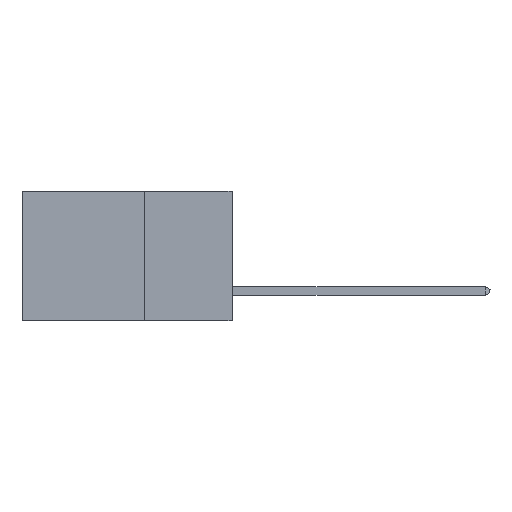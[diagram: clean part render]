
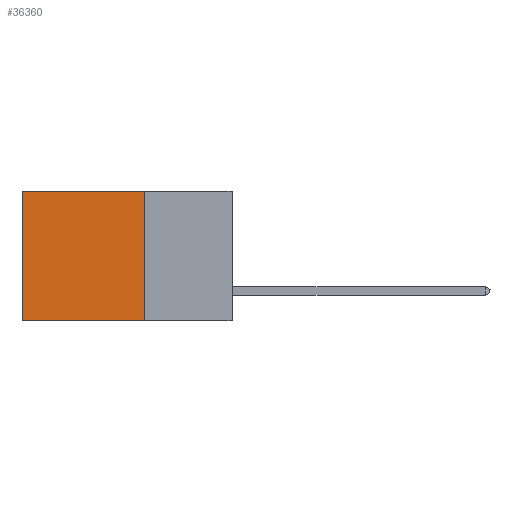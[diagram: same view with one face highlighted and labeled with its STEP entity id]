
A CAD part, left-side view. The second image highlights one B-rep face of the part: STEP entity #36360.
In plain terms, the highlighted planar face has unit normal (-1, 0, 0).
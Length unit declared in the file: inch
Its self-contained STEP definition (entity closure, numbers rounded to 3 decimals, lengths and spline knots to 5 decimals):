
#515 = VERTEX_POINT ( 'NONE', #26732 ) ;
#2666 = AXIS2_PLACEMENT_3D ( 'NONE', #9501, #15862, #3393 ) ;
#3393 = DIRECTION ( 'NONE',  ( 0., 0., -1. ) ) ;
#4523 = CARTESIAN_POINT ( 'NONE',  ( 0.2875, 0.6, 0. ) ) ;
#5504 = CARTESIAN_POINT ( 'NONE',  ( 0.2875, 0.6, 0. ) ) ;
#6185 = ORIENTED_EDGE ( 'NONE', *, *, #25124, .F. ) ;
#7430 = ORIENTED_EDGE ( 'NONE', *, *, #37695, .T. ) ;
#7458 = DIRECTION ( 'NONE',  ( 0., 1., 0. ) ) ;
#8058 = VECTOR ( 'NONE', #35329, 39.37008 ) ;
#8896 = VERTEX_POINT ( 'NONE', #17218 ) ;
#9501 = CARTESIAN_POINT ( 'NONE',  ( 0.2875, 0.25, 0. ) ) ;
#10420 = EDGE_CURVE ( 'NONE', #8896, #35351, #26040, .T. ) ;
#12358 = DIRECTION ( 'NONE',  ( 0., 1., 0. ) ) ;
#14350 = LINE ( 'NONE', #4523, #8058 ) ;
#14422 = CARTESIAN_POINT ( 'NONE',  ( 0.2875, 0.25, -0.37 ) ) ;
#15862 = DIRECTION ( 'NONE',  ( 1., 0., 0. ) ) ;
#16552 = LINE ( 'NONE', #22117, #19938 ) ;
#16942 = CARTESIAN_POINT ( 'NONE',  ( 0.2875, 0.25, -0.37 ) ) ;
#17218 = CARTESIAN_POINT ( 'NONE',  ( 0.2875, 0.25, 0. ) ) ;
#17543 = EDGE_LOOP ( 'NONE', ( #24329, #6185, #28515, #7430 ) ) ;
#19293 = LINE ( 'NONE', #16942, #31874 ) ;
#19938 = VECTOR ( 'NONE', #12358, 39.37008 ) ;
#21023 = EDGE_CURVE ( 'NONE', #31715, #515, #14350, .T. ) ;
#22117 = CARTESIAN_POINT ( 'NONE',  ( 0.2875, 0.25, 0. ) ) ;
#22353 = PLANE ( 'NONE',  #2666 ) ;
#24329 = ORIENTED_EDGE ( 'NONE', *, *, #21023, .T. ) ;
#25124 = EDGE_CURVE ( 'NONE', #35351, #515, #19293, .T. ) ;
#26040 = LINE ( 'NONE', #28101, #28966 ) ;
#26732 = CARTESIAN_POINT ( 'NONE',  ( 0.2875, 0.6, -0.37 ) ) ;
#28101 = CARTESIAN_POINT ( 'NONE',  ( 0.2875, 0.25, 0. ) ) ;
#28515 = ORIENTED_EDGE ( 'NONE', *, *, #10420, .F. ) ;
#28966 = VECTOR ( 'NONE', #31189, 39.37008 ) ;
#31189 = DIRECTION ( 'NONE',  ( 0., 0., -1. ) ) ;
#31715 = VERTEX_POINT ( 'NONE', #5504 ) ;
#31874 = VECTOR ( 'NONE', #7458, 39.37008 ) ;
#33660 = FACE_OUTER_BOUND ( 'NONE', #17543, .T. ) ;
#35329 = DIRECTION ( 'NONE',  ( 0., 0., -1. ) ) ;
#35351 = VERTEX_POINT ( 'NONE', #14422 ) ;
#36360 = ADVANCED_FACE ( 'NONE', ( #33660 ), #22353, .F. ) ;
#37695 = EDGE_CURVE ( 'NONE', #8896, #31715, #16552, .T. ) ;
